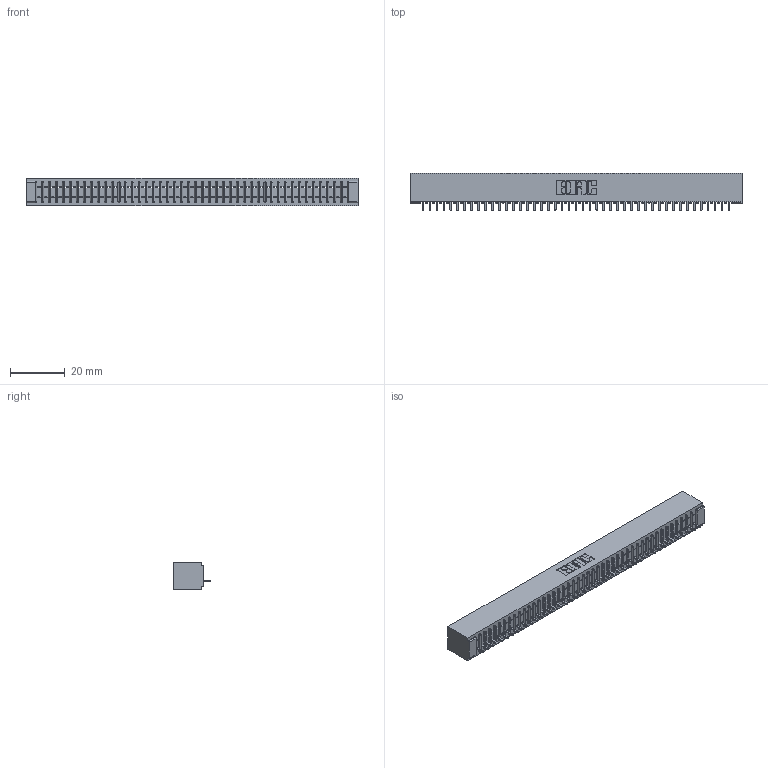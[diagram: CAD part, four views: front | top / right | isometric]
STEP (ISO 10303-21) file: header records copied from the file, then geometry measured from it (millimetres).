
FILE_DESCRIPTION (( 'STEP AP203' ), '1' );
FILE_NAME ('391-045-524-101.STEP', '2018-08-09T02:59:16', ( '' ), ( '' ), 'SwSTEP 2.0', 'SolidWorks 2016', '' );
FILE_SCHEMA (( 'CONFIG_CONTROL_DESIGN' ));
Length unit declared in the file: inch
Products named in the file (3): 341 Part_No Mounting Lugs; 341-292-001_341-292-124; 391-045-524-101
Assembly tree (46 placements, depth 2):
  391-045-524-101
    341 Part_No Mounting Lugs
    341-292-001_341-292-124  x45
Bounding box: 121.28 x 13.64 x 10.16 mm (x, y, z)
Volume: 8868.5 mm3; surface area: 14172.1 mm2
Topology: 46 solids, 46 shells, 3798 faces, 10957 edges, 7030 vertices
Faces by surface type: plane 2359, cylinder 1259, sphere 92, torus 88
Entity records: 52342 total; most frequent: CARTESIAN_POINT 8894, ORIENTED_EDGE 8882, DIRECTION 8581, EDGE_CURVE 4441, VECTOR 3595, LINE 3595, VERTEX_POINT 2806, AXIS2_PLACEMENT_3D 2493
